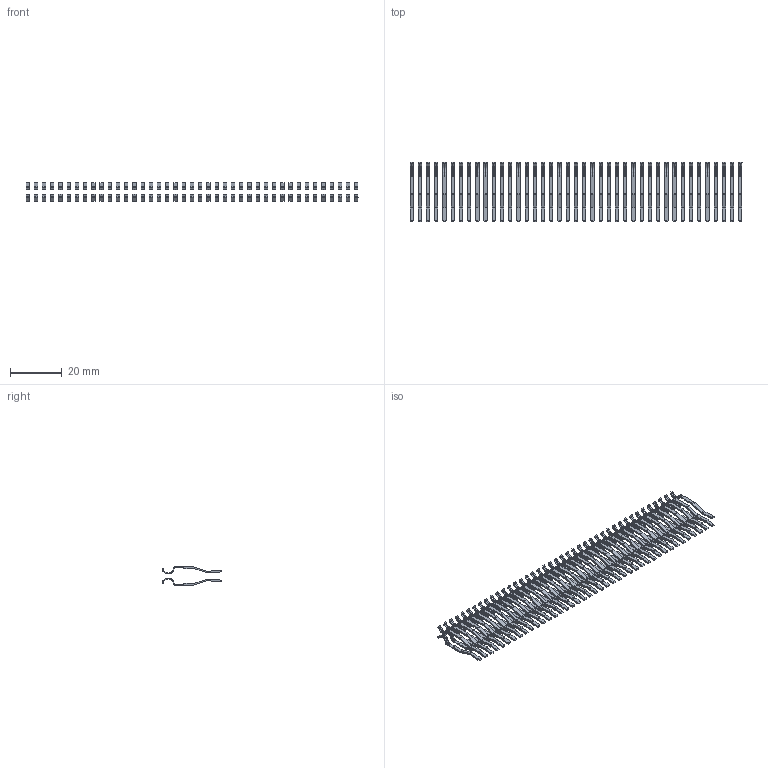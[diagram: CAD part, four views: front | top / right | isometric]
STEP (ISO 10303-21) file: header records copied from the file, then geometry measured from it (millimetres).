
FILE_DESCRIPTION (( 'STEP AP203' ), '1' );
FILE_NAME ('346-082-560-212.STEP', '2018-08-29T10:28:43', ( '' ), ( '' ), 'SwSTEP 2.0', 'SolidWorks 2016', '' );
FILE_SCHEMA (( 'CONFIG_CONTROL_DESIGN' ));
Length unit declared in the file: inch
Products named in the file (3): 345-292-001_560 Tail; 346-082-560-212; 346 Part_Flush Mounting Lugs - Side Mount
Assembly tree (83 placements, depth 2):
  346-082-560-212
    346 Part_Flush Mounting Lugs - Side Mount
    345-292-001_560 Tail  x82
Bounding box: 128.27 x 22.87 x 6.99 mm (x, y, z)
Volume: 1275.3 mm3; surface area: 7442.5 mm2
Topology: 82 solids, 82 shells, 3936 faces, 11480 edges, 7544 vertices
Faces by surface type: plane 2460, cylinder 1476
Entity records: 26983 total; most frequent: CARTESIAN_POINT 4448, ORIENTED_EDGE 4382, DIRECTION 3975, EDGE_CURVE 2191, LINE 1891, VECTOR 1891, VERTEX_POINT 1458, AXIS2_PLACEMENT_3D 1042
